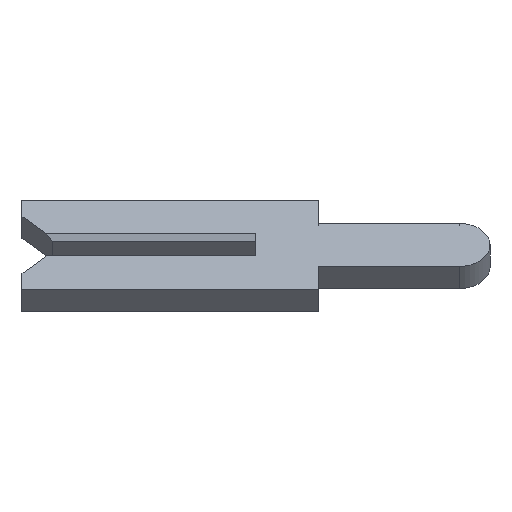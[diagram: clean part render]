
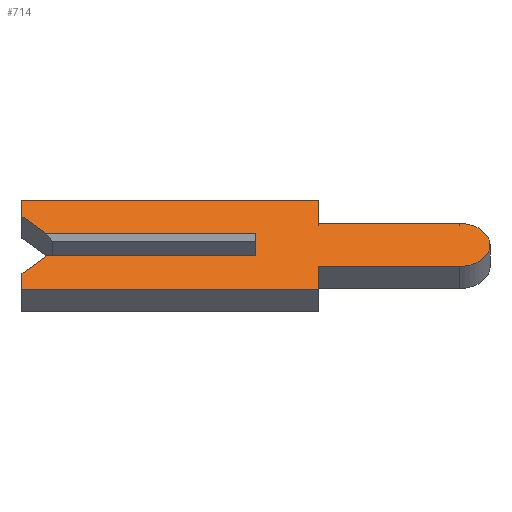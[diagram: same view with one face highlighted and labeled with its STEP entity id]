
A CAD part, left-side view. The second image highlights one B-rep face of the part: STEP entity #714.
In plain terms, the highlighted face is planar.
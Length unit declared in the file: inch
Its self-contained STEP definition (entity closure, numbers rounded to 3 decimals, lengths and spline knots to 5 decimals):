
#1 = ORIENTED_EDGE ( 'NONE', *, *, #493, .T. ) ;
#21 = VECTOR ( 'NONE', #657, 39.37008 ) ;
#26 = CARTESIAN_POINT ( 'NONE',  ( -0.01, -0.04, 0.04 ) ) ;
#57 = VECTOR ( 'NONE', #82, 39.37008 ) ;
#67 = EDGE_CURVE ( 'NONE', #116, #968, #764, .T. ) ;
#73 = EDGE_LOOP ( 'NONE', ( #1, #470, #1041, #826, #226, #558, #213, #656, #154, #501, #407, #916, #740, #599 ) ) ;
#75 = VECTOR ( 'NONE', #716, 39.37008 ) ;
#76 = PLANE ( 'NONE',  #356 ) ;
#80 = CARTESIAN_POINT ( 'NONE',  ( -0.01, 0.15, -0.04 ) ) ;
#82 = DIRECTION ( 'NONE',  ( 0., 1., 0. ) ) ;
#93 = CARTESIAN_POINT ( 'NONE',  ( -0.01, -0.04, -0.0195 ) ) ;
#97 = DIRECTION ( 'NONE',  ( 0., -0.707, 0.707 ) ) ;
#109 = LINE ( 'NONE', #670, #922 ) ;
#116 = VERTEX_POINT ( 'NONE', #442 ) ;
#126 = VECTOR ( 'NONE', #348, 39.37008 ) ;
#130 = LINE ( 'NONE', #699, #738 ) ;
#152 = VECTOR ( 'NONE', #404, 39.37008 ) ;
#154 = ORIENTED_EDGE ( 'NONE', *, *, #654, .F. ) ;
#161 = LINE ( 'NONE', #895, #176 ) ;
#163 = DIRECTION ( 'NONE',  ( 0., 0., -1. ) ) ;
#174 = DIRECTION ( 'NONE',  ( 1., 0., 0. ) ) ;
#176 = VECTOR ( 'NONE', #979, 39.37008 ) ;
#188 = CARTESIAN_POINT ( 'NONE',  ( -0.01, 0.1305, -0.0065 ) ) ;
#192 = CARTESIAN_POINT ( 'NONE',  ( -0.01, 0.134, -0.01 ) ) ;
#194 = CIRCLE ( 'NONE', #815, 0.0195 ) ;
#205 = CARTESIAN_POINT ( 'NONE',  ( -0.01, 0.15, 0.026 ) ) ;
#211 = DIRECTION ( 'NONE',  ( 0., 0., 1. ) ) ;
#213 = ORIENTED_EDGE ( 'NONE', *, *, #243, .F. ) ;
#226 = ORIENTED_EDGE ( 'NONE', *, *, #256, .F. ) ;
#238 = LINE ( 'NONE', #80, #512 ) ;
#243 = EDGE_CURVE ( 'NONE', #802, #292, #349, .T. ) ;
#248 = EDGE_CURVE ( 'NONE', #628, #879, #249, .T. ) ;
#249 = LINE ( 'NONE', #612, #336 ) ;
#255 = DIRECTION ( 'NONE',  ( 0., -1., 0. ) ) ;
#256 = EDGE_CURVE ( 'NONE', #419, #116, #130, .T. ) ;
#268 = CARTESIAN_POINT ( 'NONE',  ( -0.01, -0.04, 0.0195 ) ) ;
#284 = LINE ( 'NONE', #669, #57 ) ;
#292 = VERTEX_POINT ( 'NONE', #531 ) ;
#319 = CARTESIAN_POINT ( 'NONE',  ( -0.01, -0.1305, -0.01 ) ) ;
#326 = VERTEX_POINT ( 'NONE', #552 ) ;
#334 = CARTESIAN_POINT ( 'NONE',  ( -0.01, -0.1305, 0. ) ) ;
#336 = VECTOR ( 'NONE', #804, 39.37008 ) ;
#348 = DIRECTION ( 'NONE',  ( 0., -1., 0. ) ) ;
#349 = LINE ( 'NONE', #727, #542 ) ;
#356 = AXIS2_PLACEMENT_3D ( 'NONE', #829, #502, #163 ) ;
#404 = DIRECTION ( 'NONE',  ( 0., -1., 0. ) ) ;
#407 = ORIENTED_EDGE ( 'NONE', *, *, #601, .F. ) ;
#414 = CARTESIAN_POINT ( 'NONE',  ( -0.01, 0., -0.01 ) ) ;
#415 = EDGE_CURVE ( 'NONE', #776, #326, #161, .T. ) ;
#419 = VERTEX_POINT ( 'NONE', #564 ) ;
#442 = CARTESIAN_POINT ( 'NONE',  ( -0.01, 0.15, -0.026 ) ) ;
#462 = EDGE_CURVE ( 'NONE', #968, #628, #593, .T. ) ;
#470 = ORIENTED_EDGE ( 'NONE', *, *, #248, .F. ) ;
#492 = DIRECTION ( 'NONE',  ( 0., 0., -1. ) ) ;
#493 = EDGE_CURVE ( 'NONE', #776, #879, #906, .T. ) ;
#501 = ORIENTED_EDGE ( 'NONE', *, *, #892, .F. ) ;
#502 = DIRECTION ( 'NONE',  ( 1., 0., 0. ) ) ;
#512 = VECTOR ( 'NONE', #675, 39.37008 ) ;
#527 = CARTESIAN_POINT ( 'NONE',  ( -0.01, -0.1305, -0.0195 ) ) ;
#531 = CARTESIAN_POINT ( 'NONE',  ( -0.01, -0.04, -0.04 ) ) ;
#542 = VECTOR ( 'NONE', #783, 39.37008 ) ;
#552 = CARTESIAN_POINT ( 'NONE',  ( -0.01, 0.15, 0.026 ) ) ;
#558 = ORIENTED_EDGE ( 'NONE', *, *, #647, .F. ) ;
#563 = LINE ( 'NONE', #205, #75 ) ;
#564 = CARTESIAN_POINT ( 'NONE',  ( -0.01, 0.15, -0.04 ) ) ;
#586 = VERTEX_POINT ( 'NONE', #900 ) ;
#590 = EDGE_CURVE ( 'NONE', #326, #813, #563, .T. ) ;
#593 = LINE ( 'NONE', #319, #152 ) ;
#599 = ORIENTED_EDGE ( 'NONE', *, *, #415, .F. ) ;
#601 = EDGE_CURVE ( 'NONE', #869, #586, #109, .T. ) ;
#612 = CARTESIAN_POINT ( 'NONE',  ( -0.01, 0., 0.0065 ) ) ;
#628 = VERTEX_POINT ( 'NONE', #414 ) ;
#647 = EDGE_CURVE ( 'NONE', #292, #419, #238, .T. ) ;
#654 = EDGE_CURVE ( 'NONE', #988, #788, #194, .T. ) ;
#656 = ORIENTED_EDGE ( 'NONE', *, *, #683, .F. ) ;
#657 = DIRECTION ( 'NONE',  ( 0., -1., 0. ) ) ;
#659 = EDGE_CURVE ( 'NONE', #813, #869, #797, .T. ) ;
#669 = CARTESIAN_POINT ( 'NONE',  ( -0.01, -0.04, -0.0195 ) ) ;
#670 = CARTESIAN_POINT ( 'NONE',  ( -0.01, -0.04, 0.04 ) ) ;
#675 = DIRECTION ( 'NONE',  ( 0., 1., 0. ) ) ;
#683 = EDGE_CURVE ( 'NONE', #788, #802, #284, .T. ) ;
#687 = CARTESIAN_POINT ( 'NONE',  ( -0.01, 0., 0.01 ) ) ;
#694 = CARTESIAN_POINT ( 'NONE',  ( -0.01, 0.15, 0.04 ) ) ;
#699 = CARTESIAN_POINT ( 'NONE',  ( -0.01, 0.15, -0.026 ) ) ;
#714 = ADVANCED_FACE ( 'NONE', ( #933 ), #76, .F. ) ;
#716 = DIRECTION ( 'NONE',  ( 0., 0., 1. ) ) ;
#727 = CARTESIAN_POINT ( 'NONE',  ( -0.01, -0.04, -0.04 ) ) ;
#738 = VECTOR ( 'NONE', #211, 39.37008 ) ;
#740 = ORIENTED_EDGE ( 'NONE', *, *, #590, .F. ) ;
#746 = CARTESIAN_POINT ( 'NONE',  ( -0.01, 0.15, 0.04 ) ) ;
#749 = VECTOR ( 'NONE', #255, 39.37008 ) ;
#764 = LINE ( 'NONE', #188, #1028 ) ;
#767 = CARTESIAN_POINT ( 'NONE',  ( -0.01, -0.1305, 0.0195 ) ) ;
#776 = VERTEX_POINT ( 'NONE', #1016 ) ;
#783 = DIRECTION ( 'NONE',  ( 0., 0., -1. ) ) ;
#788 = VERTEX_POINT ( 'NONE', #527 ) ;
#797 = LINE ( 'NONE', #746, #749 ) ;
#802 = VERTEX_POINT ( 'NONE', #93 ) ;
#804 = DIRECTION ( 'NONE',  ( 0., 0., 1. ) ) ;
#813 = VERTEX_POINT ( 'NONE', #694 ) ;
#815 = AXIS2_PLACEMENT_3D ( 'NONE', #334, #174, #492 ) ;
#826 = ORIENTED_EDGE ( 'NONE', *, *, #67, .F. ) ;
#829 = CARTESIAN_POINT ( 'NONE',  ( -0.01, -0.1305, 0. ) ) ;
#832 = LINE ( 'NONE', #268, #126 ) ;
#869 = VERTEX_POINT ( 'NONE', #26 ) ;
#879 = VERTEX_POINT ( 'NONE', #687 ) ;
#892 = EDGE_CURVE ( 'NONE', #586, #988, #832, .T. ) ;
#895 = CARTESIAN_POINT ( 'NONE',  ( -0.01, 0.1305, 0.0065 ) ) ;
#900 = CARTESIAN_POINT ( 'NONE',  ( -0.01, -0.04, 0.0195 ) ) ;
#906 = LINE ( 'NONE', #1050, #21 ) ;
#916 = ORIENTED_EDGE ( 'NONE', *, *, #659, .F. ) ;
#922 = VECTOR ( 'NONE', #983, 39.37008 ) ;
#933 = FACE_OUTER_BOUND ( 'NONE', #73, .T. ) ;
#968 = VERTEX_POINT ( 'NONE', #192 ) ;
#979 = DIRECTION ( 'NONE',  ( 0., 0.707, 0.707 ) ) ;
#983 = DIRECTION ( 'NONE',  ( 0., 0., -1. ) ) ;
#988 = VERTEX_POINT ( 'NONE', #767 ) ;
#1016 = CARTESIAN_POINT ( 'NONE',  ( -0.01, 0.134, 0.01 ) ) ;
#1028 = VECTOR ( 'NONE', #97, 39.37008 ) ;
#1041 = ORIENTED_EDGE ( 'NONE', *, *, #462, .F. ) ;
#1050 = CARTESIAN_POINT ( 'NONE',  ( -0.01, 0.15, 0.01 ) ) ;
